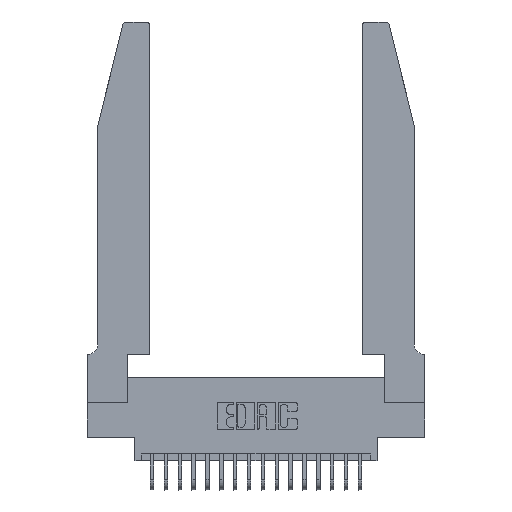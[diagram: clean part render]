
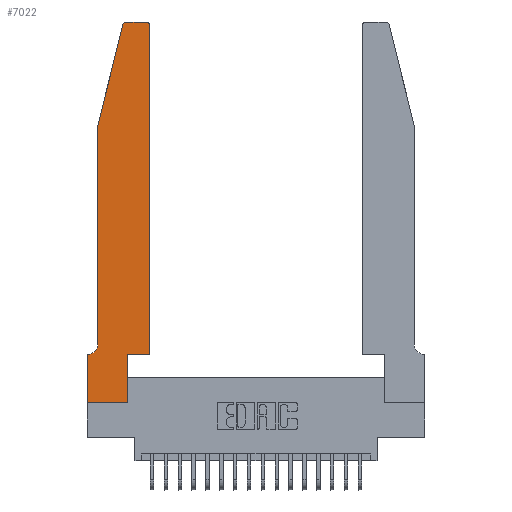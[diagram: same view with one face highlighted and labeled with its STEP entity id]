
A CAD part, top view. The second image highlights one B-rep face of the part: STEP entity #7022.
In plain terms, the highlighted planar face has unit normal (0, 0, 1).
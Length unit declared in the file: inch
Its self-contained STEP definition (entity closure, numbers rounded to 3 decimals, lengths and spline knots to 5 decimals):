
#54 = CARTESIAN_POINT ( 'NONE',  ( 0.25487, 2.72718, 0.37 ) ) ;
#395 = ORIENTED_EDGE ( 'NONE', *, *, #16260, .T. ) ;
#437 = ORIENTED_EDGE ( 'NONE', *, *, #20073, .T. ) ;
#665 = CIRCLE ( 'NONE', #11448, 0.03 ) ;
#700 = CARTESIAN_POINT ( 'NONE',  ( 0., 0., 0.37 ) ) ;
#706 = CIRCLE ( 'NONE', #16856, 0.03 ) ;
#1198 = DIRECTION ( 'NONE',  ( 1., 0., 0. ) ) ;
#1274 = CARTESIAN_POINT ( 'NONE',  ( 0.0055, 0.42, 0.37 ) ) ;
#1577 = EDGE_CURVE ( 'NONE', #14424, #7029, #706, .T. ) ;
#1643 = LINE ( 'NONE', #10598, #15084 ) ;
#1692 = CARTESIAN_POINT ( 'NONE',  ( 0.4205, 2.75, 0.37 ) ) ;
#1798 = CARTESIAN_POINT ( 'NONE',  ( 0., 0.35, 0.37 ) ) ;
#2533 = DIRECTION ( 'NONE',  ( 1., 0., 0. ) ) ;
#2656 = EDGE_CURVE ( 'NONE', #7029, #3982, #18702, .T. ) ;
#2693 = EDGE_CURVE ( 'NONE', #3982, #4438, #9556, .T. ) ;
#3009 = CARTESIAN_POINT ( 'NONE',  ( 0.2865, 0.35, 0.37 ) ) ;
#3101 = DIRECTION ( 'NONE',  ( -1., 0., 0. ) ) ;
#3107 = CARTESIAN_POINT ( 'NONE',  ( 0.0755, 2., 0.37 ) ) ;
#3221 = CARTESIAN_POINT ( 'NONE',  ( 0.2605, 2.75, 0.37 ) ) ;
#3528 = ORIENTED_EDGE ( 'NONE', *, *, #2693, .T. ) ;
#3651 = DIRECTION ( 'NONE',  ( 1., 0., 0. ) ) ;
#3982 = VERTEX_POINT ( 'NONE', #15344 ) ;
#4438 = VERTEX_POINT ( 'NONE', #21638 ) ;
#4594 = EDGE_CURVE ( 'NONE', #4438, #19433, #22442, .T. ) ;
#4870 = VECTOR ( 'NONE', #8421, 39.37008 ) ;
#4916 = DIRECTION ( 'NONE',  ( -1., 0., 0. ) ) ;
#5024 = VERTEX_POINT ( 'NONE', #16411 ) ;
#5033 = DIRECTION ( 'NONE',  ( 0., -1., 0. ) ) ;
#5106 = CARTESIAN_POINT ( 'NONE',  ( 0.2865, 0., 0.37 ) ) ;
#6247 = ORIENTED_EDGE ( 'NONE', *, *, #2656, .T. ) ;
#6306 = DIRECTION ( 'NONE',  ( 0., 1., 0. ) ) ;
#6907 = DIRECTION ( 'NONE',  ( 0., 1., 0. ) ) ;
#7022 = ADVANCED_FACE ( 'NONE', ( #10383 ), #7168, .T. ) ;
#7029 = VERTEX_POINT ( 'NONE', #54 ) ;
#7141 = ORIENTED_EDGE ( 'NONE', *, *, #11781, .T. ) ;
#7147 = CARTESIAN_POINT ( 'NONE',  ( 0.0055, 0.35, 0.37 ) ) ;
#7168 = PLANE ( 'NONE',  #14643 ) ;
#7291 = ORIENTED_EDGE ( 'NONE', *, *, #4594, .T. ) ;
#7609 = LINE ( 'NONE', #3221, #16268 ) ;
#8169 = EDGE_CURVE ( 'NONE', #18893, #19710, #21369, .T. ) ;
#8421 = DIRECTION ( 'NONE',  ( -0.239, -0.971, 0. ) ) ;
#8429 = VECTOR ( 'NONE', #2533, 39.37008 ) ;
#8450 = VECTOR ( 'NONE', #5033, 39.37008 ) ;
#8923 = DIRECTION ( 'NONE',  ( 1., 0., 0. ) ) ;
#9175 = CARTESIAN_POINT ( 'NONE',  ( 0.284, 2.75, 0.37 ) ) ;
#9556 = LINE ( 'NONE', #13742, #8450 ) ;
#9584 = CARTESIAN_POINT ( 'NONE',  ( 0.4505, 2.72, 0.37 ) ) ;
#10182 = VERTEX_POINT ( 'NONE', #1692 ) ;
#10190 = EDGE_CURVE ( 'NONE', #12800, #5024, #1643, .T. ) ;
#10252 = ORIENTED_EDGE ( 'NONE', *, *, #1577, .T. ) ;
#10322 = LINE ( 'NONE', #13057, #14356 ) ;
#10383 = FACE_OUTER_BOUND ( 'NONE', #14141, .T. ) ;
#10479 = LINE ( 'NONE', #22455, #15044 ) ;
#10598 = CARTESIAN_POINT ( 'NONE',  ( 0., 0., 0.37 ) ) ;
#10692 = VERTEX_POINT ( 'NONE', #3009 ) ;
#10794 = VERTEX_POINT ( 'NONE', #5106 ) ;
#10920 = LINE ( 'NONE', #17461, #19509 ) ;
#11024 = ORIENTED_EDGE ( 'NONE', *, *, #8169, .T. ) ;
#11448 = AXIS2_PLACEMENT_3D ( 'NONE', #22086, #11782, #1198 ) ;
#11669 = VECTOR ( 'NONE', #6306, 39.37008 ) ;
#11781 = EDGE_CURVE ( 'NONE', #10794, #10692, #10479, .T. ) ;
#11782 = DIRECTION ( 'NONE',  ( 0., 0., 1. ) ) ;
#12105 = ORIENTED_EDGE ( 'NONE', *, *, #15710, .T. ) ;
#12510 = DIRECTION ( 'NONE',  ( 0., 0., 1. ) ) ;
#12800 = VERTEX_POINT ( 'NONE', #22044 ) ;
#13057 = CARTESIAN_POINT ( 'NONE',  ( 0.0755, 0.35, 0.37 ) ) ;
#13587 = DIRECTION ( 'NONE',  ( 0., 0., -1. ) ) ;
#13742 = CARTESIAN_POINT ( 'NONE',  ( 0.0755, 2., 0.37 ) ) ;
#14141 = EDGE_LOOP ( 'NONE', ( #14611, #10252, #6247, #3528, #7291, #17567, #21224, #395, #7141, #437, #11024, #12105 ) ) ;
#14356 = VECTOR ( 'NONE', #14779, 39.37008 ) ;
#14424 = VERTEX_POINT ( 'NONE', #9175 ) ;
#14611 = ORIENTED_EDGE ( 'NONE', *, *, #16509, .T. ) ;
#14643 = AXIS2_PLACEMENT_3D ( 'NONE', #1798, #19244, #8923 ) ;
#14779 = DIRECTION ( 'NONE',  ( -1., 0., 0. ) ) ;
#15044 = VECTOR ( 'NONE', #6907, 39.37008 ) ;
#15084 = VECTOR ( 'NONE', #22611, 39.37008 ) ;
#15095 = CARTESIAN_POINT ( 'NONE',  ( 0.4505, 0.35, 0.37 ) ) ;
#15336 = AXIS2_PLACEMENT_3D ( 'NONE', #1274, #13587, #3101 ) ;
#15344 = CARTESIAN_POINT ( 'NONE',  ( 0.0755, 2., 0.37 ) ) ;
#15690 = CARTESIAN_POINT ( 'NONE',  ( 0.4505, 0.35, 0.37 ) ) ;
#15710 = EDGE_CURVE ( 'NONE', #19710, #10182, #665, .T. ) ;
#16260 = EDGE_CURVE ( 'NONE', #5024, #10794, #22207, .T. ) ;
#16268 = VECTOR ( 'NONE', #4916, 39.37008 ) ;
#16411 = CARTESIAN_POINT ( 'NONE',  ( 0., 0., 0.37 ) ) ;
#16509 = EDGE_CURVE ( 'NONE', #10182, #14424, #7609, .T. ) ;
#16856 = AXIS2_PLACEMENT_3D ( 'NONE', #18508, #12510, #19460 ) ;
#17461 = CARTESIAN_POINT ( 'NONE',  ( 0.4505, 0.35, 0.37 ) ) ;
#17567 = ORIENTED_EDGE ( 'NONE', *, *, #22260, .T. ) ;
#18508 = CARTESIAN_POINT ( 'NONE',  ( 0.284, 2.72, 0.37 ) ) ;
#18702 = LINE ( 'NONE', #3107, #4870 ) ;
#18893 = VERTEX_POINT ( 'NONE', #15095 ) ;
#19244 = DIRECTION ( 'NONE',  ( 0., 0., 1. ) ) ;
#19433 = VERTEX_POINT ( 'NONE', #7147 ) ;
#19460 = DIRECTION ( 'NONE',  ( 1., 0., 0. ) ) ;
#19509 = VECTOR ( 'NONE', #3651, 39.37008 ) ;
#19710 = VERTEX_POINT ( 'NONE', #9584 ) ;
#20073 = EDGE_CURVE ( 'NONE', #10692, #18893, #10920, .T. ) ;
#21224 = ORIENTED_EDGE ( 'NONE', *, *, #10190, .T. ) ;
#21369 = LINE ( 'NONE', #15690, #11669 ) ;
#21638 = CARTESIAN_POINT ( 'NONE',  ( 0.0755, 0.42, 0.37 ) ) ;
#22044 = CARTESIAN_POINT ( 'NONE',  ( 0., 0.35, 0.37 ) ) ;
#22086 = CARTESIAN_POINT ( 'NONE',  ( 0.4205, 2.72, 0.37 ) ) ;
#22207 = LINE ( 'NONE', #700, #8429 ) ;
#22260 = EDGE_CURVE ( 'NONE', #19433, #12800, #10322, .T. ) ;
#22442 = CIRCLE ( 'NONE', #15336, 0.07 ) ;
#22455 = CARTESIAN_POINT ( 'NONE',  ( 0.2865, 0.35, 0.37 ) ) ;
#22611 = DIRECTION ( 'NONE',  ( 0., -1., 0. ) ) ;
